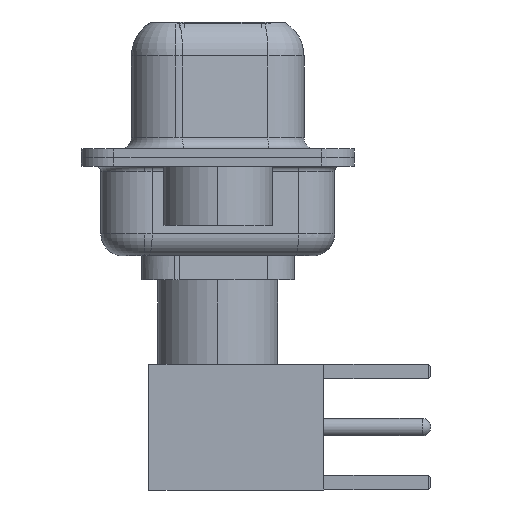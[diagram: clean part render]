
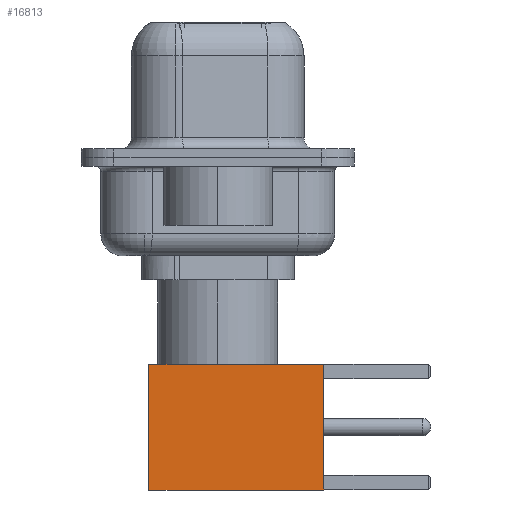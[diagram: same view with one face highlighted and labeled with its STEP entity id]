
A CAD part, left-side view. The second image highlights one B-rep face of the part: STEP entity #16813.
In plain terms, the highlighted face is planar.
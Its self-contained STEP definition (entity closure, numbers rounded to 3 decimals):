
#120 = VECTOR ( 'NONE', #16443, 1000. ) ;
#1326 = VERTEX_POINT ( 'NONE', #11411 ) ;
#2202 = EDGE_CURVE ( 'NONE', #1326, #5545, #10888, .T. ) ;
#2564 = FACE_OUTER_BOUND ( 'NONE', #16923, .T. ) ;
#3760 = PLANE ( 'NONE',  #13625 ) ;
#4998 = CARTESIAN_POINT ( 'NONE',  ( 0., 2.875, 8. ) ) ;
#5446 = CARTESIAN_POINT ( 'NONE',  ( -2.875, 2.875, 0. ) ) ;
#5528 = LINE ( 'NONE', #15791, #5584 ) ;
#5545 = VERTEX_POINT ( 'NONE', #5446 ) ;
#5584 = VECTOR ( 'NONE', #7394, 1000. ) ;
#6161 = VERTEX_POINT ( 'NONE', #8861 ) ;
#6777 = ORIENTED_EDGE ( 'NONE', *, *, #14104, .T. ) ;
#6861 = DIRECTION ( 'NONE',  ( 0., 0., 1. ) ) ;
#7394 = DIRECTION ( 'NONE',  ( 0., 0., -1. ) ) ;
#8861 = CARTESIAN_POINT ( 'NONE',  ( 2.875, 2.875, 8. ) ) ;
#9951 = ORIENTED_EDGE ( 'NONE', *, *, #2202, .F. ) ;
#10650 = CARTESIAN_POINT ( 'NONE',  ( 0., 2.875, 0. ) ) ;
#10692 = DIRECTION ( 'NONE',  ( -1., 0., 0. ) ) ;
#10888 = LINE ( 'NONE', #16216, #13613 ) ;
#11411 = CARTESIAN_POINT ( 'NONE',  ( -2.875, 2.875, 8. ) ) ;
#13613 = VECTOR ( 'NONE', #16585, 1000. ) ;
#13625 = AXIS2_PLACEMENT_3D ( 'NONE', #15154, #13954, #6861 ) ;
#13825 = EDGE_CURVE ( 'NONE', #6161, #1326, #17886, .T. ) ;
#13954 = DIRECTION ( 'NONE',  ( 0., 1., 0. ) ) ;
#14104 = EDGE_CURVE ( 'NONE', #14493, #5545, #14422, .T. ) ;
#14282 = CARTESIAN_POINT ( 'NONE',  ( 2.875, 2.875, 0. ) ) ;
#14422 = LINE ( 'NONE', #10650, #120 ) ;
#14493 = VERTEX_POINT ( 'NONE', #14282 ) ;
#15154 = CARTESIAN_POINT ( 'NONE',  ( 2.875, 2.875, 0. ) ) ;
#15521 = ORIENTED_EDGE ( 'NONE', *, *, #17596, .T. ) ;
#15791 = CARTESIAN_POINT ( 'NONE',  ( 2.875, 2.875, 0. ) ) ;
#15901 = VECTOR ( 'NONE', #10692, 1000. ) ;
#16216 = CARTESIAN_POINT ( 'NONE',  ( -2.875, 2.875, 0. ) ) ;
#16443 = DIRECTION ( 'NONE',  ( -1., 0., 0. ) ) ;
#16585 = DIRECTION ( 'NONE',  ( 0., 0., -1. ) ) ;
#16813 = ADVANCED_FACE ( 'NONE', ( #2564 ), #3760, .T. ) ;
#16923 = EDGE_LOOP ( 'NONE', ( #15521, #6777, #9951, #17954 ) ) ;
#17596 = EDGE_CURVE ( 'NONE', #6161, #14493, #5528, .T. ) ;
#17886 = LINE ( 'NONE', #4998, #15901 ) ;
#17954 = ORIENTED_EDGE ( 'NONE', *, *, #13825, .F. ) ;
